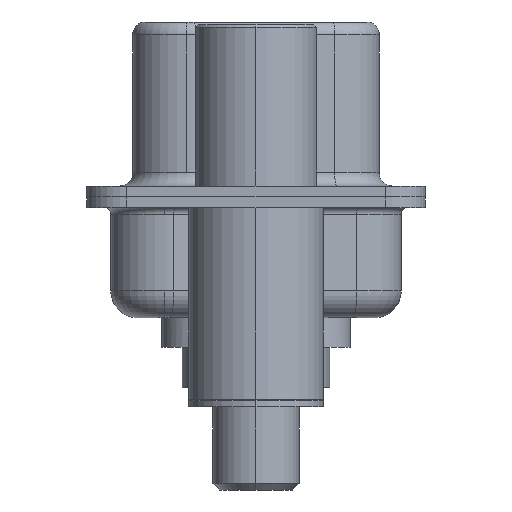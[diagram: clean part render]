
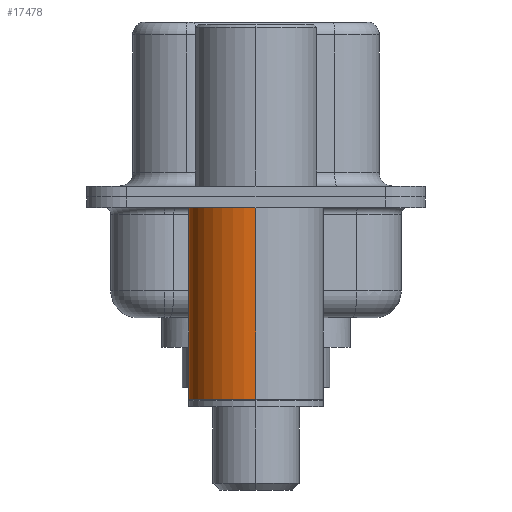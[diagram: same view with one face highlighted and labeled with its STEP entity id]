
A CAD part, left-side view. The second image highlights one B-rep face of the part: STEP entity #17478.
In plain terms, the highlighted cylindrical face has radius 2.5 mm (diameter 5 mm), a partial arc.
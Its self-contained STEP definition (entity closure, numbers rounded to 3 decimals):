
#67 = CIRCLE ( 'NONE', #17555, 2.5 ) ;
#288 = VERTEX_POINT ( 'NONE', #21271 ) ;
#2238 = CYLINDRICAL_SURFACE ( 'NONE', #4906, 2.5 ) ;
#2557 = CARTESIAN_POINT ( 'NONE',  ( 0., 0., -0.4 ) ) ;
#2893 = CARTESIAN_POINT ( 'NONE',  ( 0., 0., 0.581 ) ) ;
#2970 = DIRECTION ( 'NONE',  ( 1., 0., 0. ) ) ;
#3670 = ORIENTED_EDGE ( 'NONE', *, *, #21108, .F. ) ;
#3725 = ORIENTED_EDGE ( 'NONE', *, *, #17148, .T. ) ;
#4306 = DIRECTION ( 'NONE',  ( 1., 0., 0. ) ) ;
#4906 = AXIS2_PLACEMENT_3D ( 'NONE', #2893, #9995, #2970 ) ;
#5445 = DIRECTION ( 'NONE',  ( 0., 0., 1. ) ) ;
#5893 = AXIS2_PLACEMENT_3D ( 'NONE', #15992, #5445, #17692 ) ;
#6305 = CARTESIAN_POINT ( 'NONE',  ( -2.5, 0., -7.525 ) ) ;
#7116 = DIRECTION ( 'NONE',  ( 0., 0., 1. ) ) ;
#7844 = ORIENTED_EDGE ( 'NONE', *, *, #9543, .F. ) ;
#8951 = CARTESIAN_POINT ( 'NONE',  ( 2.5, 0., 0.581 ) ) ;
#9543 = EDGE_CURVE ( 'NONE', #14782, #288, #67, .T. ) ;
#9995 = DIRECTION ( 'NONE',  ( 0., 0., 1. ) ) ;
#10361 = LINE ( 'NONE', #8951, #15086 ) ;
#11150 = CIRCLE ( 'NONE', #5893, 2.5 ) ;
#11561 = FACE_OUTER_BOUND ( 'NONE', #19616, .T. ) ;
#12761 = VERTEX_POINT ( 'NONE', #13477 ) ;
#13477 = CARTESIAN_POINT ( 'NONE',  ( 2.5, 0., -7.525 ) ) ;
#13926 = EDGE_CURVE ( 'NONE', #12761, #14277, #11150, .T. ) ;
#14124 = CARTESIAN_POINT ( 'NONE',  ( -2.5, 0., 0.581 ) ) ;
#14277 = VERTEX_POINT ( 'NONE', #6305 ) ;
#14782 = VERTEX_POINT ( 'NONE', #14882 ) ;
#14859 = DIRECTION ( 'NONE',  ( 0., 0., 1. ) ) ;
#14882 = CARTESIAN_POINT ( 'NONE',  ( 2.5, 0., -0.4 ) ) ;
#15086 = VECTOR ( 'NONE', #19411, 1000. ) ;
#15985 = VECTOR ( 'NONE', #7116, 1000. ) ;
#15992 = CARTESIAN_POINT ( 'NONE',  ( 0., 0., -7.525 ) ) ;
#16093 = ORIENTED_EDGE ( 'NONE', *, *, #13926, .T. ) ;
#17148 = EDGE_CURVE ( 'NONE', #14277, #288, #20557, .T. ) ;
#17478 = ADVANCED_FACE ( 'NONE', ( #11561 ), #2238, .T. ) ;
#17555 = AXIS2_PLACEMENT_3D ( 'NONE', #2557, #14859, #4306 ) ;
#17692 = DIRECTION ( 'NONE',  ( 1., 0., 0. ) ) ;
#19411 = DIRECTION ( 'NONE',  ( 0., 0., 1. ) ) ;
#19616 = EDGE_LOOP ( 'NONE', ( #16093, #3725, #7844, #3670 ) ) ;
#20557 = LINE ( 'NONE', #14124, #15985 ) ;
#21108 = EDGE_CURVE ( 'NONE', #12761, #14782, #10361, .T. ) ;
#21271 = CARTESIAN_POINT ( 'NONE',  ( -2.5, 0., -0.4 ) ) ;
